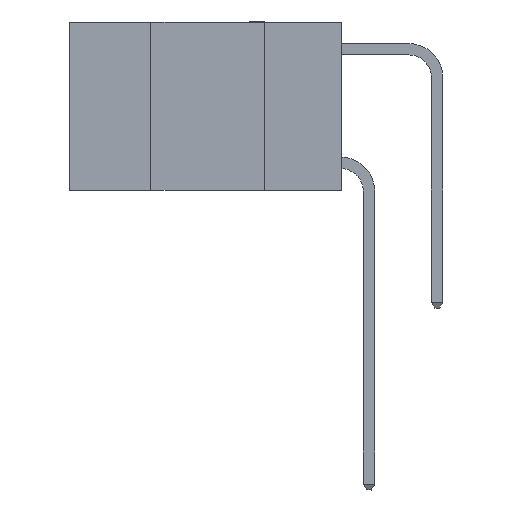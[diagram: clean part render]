
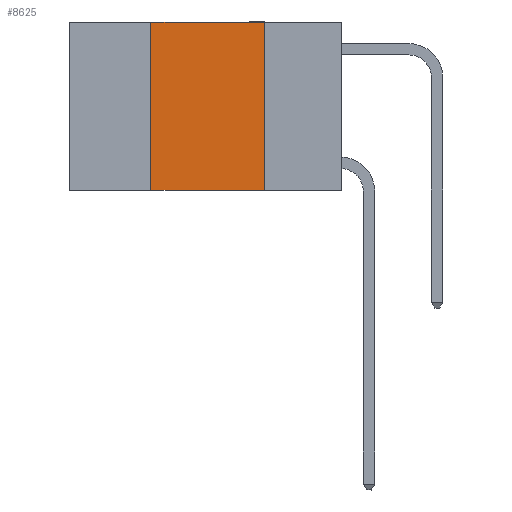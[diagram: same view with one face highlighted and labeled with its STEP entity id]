
A CAD part, left-side view. The second image highlights one B-rep face of the part: STEP entity #8625.
In plain terms, the highlighted planar face has unit normal (-1, 0, 0).
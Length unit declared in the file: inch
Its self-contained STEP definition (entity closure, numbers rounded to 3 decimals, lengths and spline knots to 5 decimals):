
#473 = LINE ( 'NONE', #15190, #7943 ) ;
#476 = CARTESIAN_POINT ( 'NONE',  ( 0., 0.17, 0. ) ) ;
#672 = VERTEX_POINT ( 'NONE', #12091 ) ;
#2119 = EDGE_CURVE ( 'NONE', #672, #14178, #12175, .T. ) ;
#2888 = ORIENTED_EDGE ( 'NONE', *, *, #14894, .F. ) ;
#2925 = ORIENTED_EDGE ( 'NONE', *, *, #4201, .F. ) ;
#3036 = ORIENTED_EDGE ( 'NONE', *, *, #2119, .T. ) ;
#3197 = CARTESIAN_POINT ( 'NONE',  ( 0., 0.17, -0.37 ) ) ;
#4071 = DIRECTION ( 'NONE',  ( 0., 0., 1. ) ) ;
#4201 = EDGE_CURVE ( 'NONE', #672, #10904, #473, .T. ) ;
#4870 = EDGE_CURVE ( 'NONE', #10904, #11993, #16404, .T. ) ;
#5697 = AXIS2_PLACEMENT_3D ( 'NONE', #6987, #16700, #8400 ) ;
#6776 = CARTESIAN_POINT ( 'NONE',  ( 0., 0.6, 0. ) ) ;
#6987 = CARTESIAN_POINT ( 'NONE',  ( 0., 0.6, 0. ) ) ;
#7943 = VECTOR ( 'NONE', #4071, 39.37008 ) ;
#8400 = DIRECTION ( 'NONE',  ( 0., 0., -1. ) ) ;
#8625 = ADVANCED_FACE ( 'NONE', ( #12105 ), #15336, .F. ) ;
#8751 = VECTOR ( 'NONE', #17095, 39.37008 ) ;
#9013 = VECTOR ( 'NONE', #16486, 39.37008 ) ;
#9355 = CARTESIAN_POINT ( 'NONE',  ( 0., 0.42, 0. ) ) ;
#10276 = ORIENTED_EDGE ( 'NONE', *, *, #4870, .F. ) ;
#10904 = VERTEX_POINT ( 'NONE', #9355 ) ;
#11993 = VERTEX_POINT ( 'NONE', #476 ) ;
#12091 = CARTESIAN_POINT ( 'NONE',  ( 0., 0.42, -0.37 ) ) ;
#12105 = FACE_OUTER_BOUND ( 'NONE', #16643, .T. ) ;
#12175 = LINE ( 'NONE', #15235, #15826 ) ;
#12502 = LINE ( 'NONE', #13003, #8751 ) ;
#13003 = CARTESIAN_POINT ( 'NONE',  ( 0., 0.17, 0. ) ) ;
#14178 = VERTEX_POINT ( 'NONE', #3197 ) ;
#14894 = EDGE_CURVE ( 'NONE', #11993, #14178, #12502, .T. ) ;
#15190 = CARTESIAN_POINT ( 'NONE',  ( 0., 0.42, 0. ) ) ;
#15235 = CARTESIAN_POINT ( 'NONE',  ( 0., 0.6, -0.37 ) ) ;
#15336 = PLANE ( 'NONE',  #5697 ) ;
#15826 = VECTOR ( 'NONE', #16609, 39.37008 ) ;
#16404 = LINE ( 'NONE', #6776, #9013 ) ;
#16486 = DIRECTION ( 'NONE',  ( 0., -1., 0. ) ) ;
#16609 = DIRECTION ( 'NONE',  ( 0., -1., 0. ) ) ;
#16643 = EDGE_LOOP ( 'NONE', ( #2888, #10276, #2925, #3036 ) ) ;
#16700 = DIRECTION ( 'NONE',  ( 1., 0., 0. ) ) ;
#17095 = DIRECTION ( 'NONE',  ( 0., 0., -1. ) ) ;
